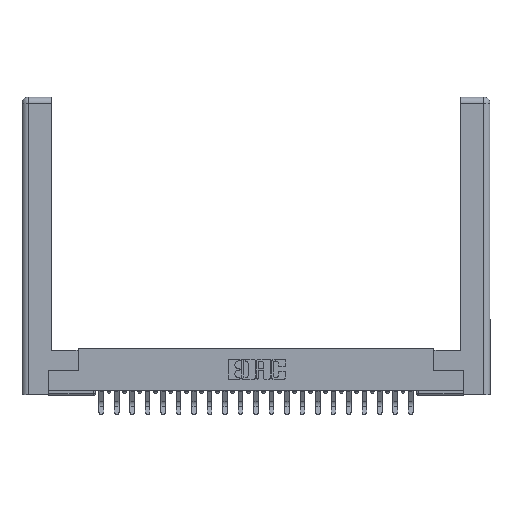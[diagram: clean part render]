
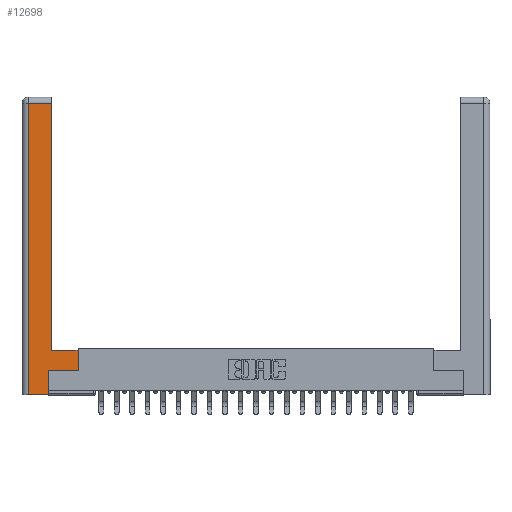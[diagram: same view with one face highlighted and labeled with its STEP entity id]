
A CAD part, top view. The second image highlights one B-rep face of the part: STEP entity #12698.
In plain terms, the highlighted planar face has unit normal (0, 0, 1).
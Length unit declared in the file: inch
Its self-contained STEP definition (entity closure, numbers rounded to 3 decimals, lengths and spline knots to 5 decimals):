
#137 = VERTEX_POINT ( 'NONE', #7672 ) ;
#222 = VECTOR ( 'NONE', #20500, 39.37008 ) ;
#310 = DIRECTION ( 'NONE',  ( -1., 0., 0. ) ) ;
#866 = CARTESIAN_POINT ( 'NONE',  ( 0.295, 0.45, 0. ) ) ;
#1529 = CARTESIAN_POINT ( 'NONE',  ( 0.265, 0.245, 0. ) ) ;
#2002 = CARTESIAN_POINT ( 'NONE',  ( 0.265, 0.245, 0. ) ) ;
#2215 = CARTESIAN_POINT ( 'NONE',  ( 0.295, 3., 0. ) ) ;
#2241 = DIRECTION ( 'NONE',  ( 0., 1., 0. ) ) ;
#2376 = CARTESIAN_POINT ( 'NONE',  ( 0.565, 0.45, 0. ) ) ;
#3333 = DIRECTION ( 'NONE',  ( -1., 0., 0. ) ) ;
#3425 = VECTOR ( 'NONE', #5353, 39.37008 ) ;
#3802 = CARTESIAN_POINT ( 'NONE',  ( 0.0615, 0., 0. ) ) ;
#4924 = VECTOR ( 'NONE', #2241, 39.37008 ) ;
#5151 = LINE ( 'NONE', #2376, #13842 ) ;
#5353 = DIRECTION ( 'NONE',  ( 1., 0., 0. ) ) ;
#6339 = DIRECTION ( 'NONE',  ( 0., 1., 0. ) ) ;
#6709 = CARTESIAN_POINT ( 'NONE',  ( 0.565, 0.245, 0. ) ) ;
#6774 = EDGE_CURVE ( 'NONE', #10623, #21197, #7191, .T. ) ;
#7162 = CARTESIAN_POINT ( 'NONE',  ( 0.0615, 0., 0. ) ) ;
#7191 = LINE ( 'NONE', #2215, #222 ) ;
#7672 = CARTESIAN_POINT ( 'NONE',  ( 0.0615, 2.94, 0. ) ) ;
#7802 = EDGE_CURVE ( 'NONE', #11105, #19521, #10933, .T. ) ;
#8065 = VERTEX_POINT ( 'NONE', #20091 ) ;
#8224 = EDGE_LOOP ( 'NONE', ( #17515, #17578, #12145, #13250, #12517, #20709, #16682, #8991 ) ) ;
#8831 = LINE ( 'NONE', #7162, #23027 ) ;
#8832 = PLANE ( 'NONE',  #16353 ) ;
#8991 = ORIENTED_EDGE ( 'NONE', *, *, #12988, .T. ) ;
#9034 = CARTESIAN_POINT ( 'NONE',  ( 0.295, 2.94, 0. ) ) ;
#9441 = EDGE_CURVE ( 'NONE', #137, #11105, #8831, .T. ) ;
#10280 = CARTESIAN_POINT ( 'NONE',  ( 0.295, 0.45, 0. ) ) ;
#10623 = VERTEX_POINT ( 'NONE', #866 ) ;
#10686 = VECTOR ( 'NONE', #310, 39.37008 ) ;
#10757 = EDGE_CURVE ( 'NONE', #15092, #19141, #20400, .T. ) ;
#10933 = LINE ( 'NONE', #20326, #3425 ) ;
#10991 = LINE ( 'NONE', #17242, #10686 ) ;
#11105 = VERTEX_POINT ( 'NONE', #3802 ) ;
#12145 = ORIENTED_EDGE ( 'NONE', *, *, #9441, .T. ) ;
#12483 = DIRECTION ( 'NONE',  ( 1., 0., 0. ) ) ;
#12517 = ORIENTED_EDGE ( 'NONE', *, *, #13322, .T. ) ;
#12698 = ADVANCED_FACE ( 'NONE', ( #14773 ), #8832, .F. ) ;
#12988 = EDGE_CURVE ( 'NONE', #8065, #10623, #18265, .T. ) ;
#13250 = ORIENTED_EDGE ( 'NONE', *, *, #7802, .T. ) ;
#13297 = VECTOR ( 'NONE', #3333, 39.37008 ) ;
#13322 = EDGE_CURVE ( 'NONE', #19521, #15092, #14778, .T. ) ;
#13842 = VECTOR ( 'NONE', #6339, 39.37008 ) ;
#14131 = EDGE_CURVE ( 'NONE', #19141, #8065, #5151, .T. ) ;
#14292 = VECTOR ( 'NONE', #12483, 39.37008 ) ;
#14373 = CARTESIAN_POINT ( 'NONE',  ( 0.565, 0.245, 0. ) ) ;
#14495 = DIRECTION ( 'NONE',  ( -1., 0., 0. ) ) ;
#14773 = FACE_OUTER_BOUND ( 'NONE', #8224, .T. ) ;
#14778 = LINE ( 'NONE', #2002, #4924 ) ;
#15092 = VERTEX_POINT ( 'NONE', #1529 ) ;
#16353 = AXIS2_PLACEMENT_3D ( 'NONE', #21794, #23744, #14495 ) ;
#16682 = ORIENTED_EDGE ( 'NONE', *, *, #14131, .T. ) ;
#17242 = CARTESIAN_POINT ( 'NONE',  ( 0.0615, 2.94, 0. ) ) ;
#17515 = ORIENTED_EDGE ( 'NONE', *, *, #6774, .T. ) ;
#17578 = ORIENTED_EDGE ( 'NONE', *, *, #22062, .T. ) ;
#18265 = LINE ( 'NONE', #10280, #13297 ) ;
#19141 = VERTEX_POINT ( 'NONE', #14373 ) ;
#19521 = VERTEX_POINT ( 'NONE', #20459 ) ;
#20091 = CARTESIAN_POINT ( 'NONE',  ( 0.565, 0.45, 0. ) ) ;
#20326 = CARTESIAN_POINT ( 'NONE',  ( 0.265, 0., 0. ) ) ;
#20400 = LINE ( 'NONE', #6709, #14292 ) ;
#20459 = CARTESIAN_POINT ( 'NONE',  ( 0.265, 0., 0. ) ) ;
#20500 = DIRECTION ( 'NONE',  ( 0., 1., 0. ) ) ;
#20709 = ORIENTED_EDGE ( 'NONE', *, *, #10757, .T. ) ;
#21197 = VERTEX_POINT ( 'NONE', #9034 ) ;
#21794 = CARTESIAN_POINT ( 'NONE',  ( 0., 0., 0. ) ) ;
#21831 = DIRECTION ( 'NONE',  ( 0., -1., 0. ) ) ;
#22062 = EDGE_CURVE ( 'NONE', #21197, #137, #10991, .T. ) ;
#23027 = VECTOR ( 'NONE', #21831, 39.37008 ) ;
#23744 = DIRECTION ( 'NONE',  ( 0., 0., -1. ) ) ;
